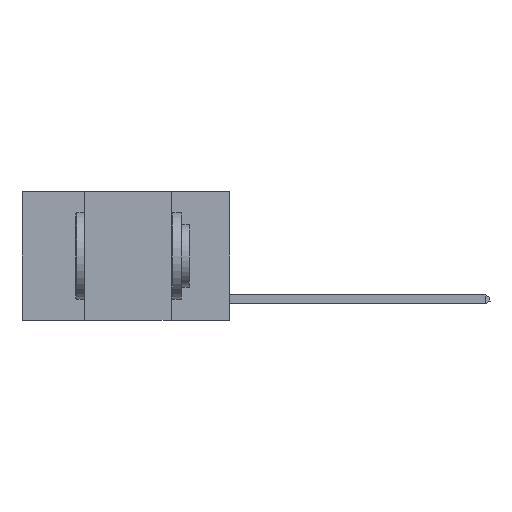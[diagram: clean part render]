
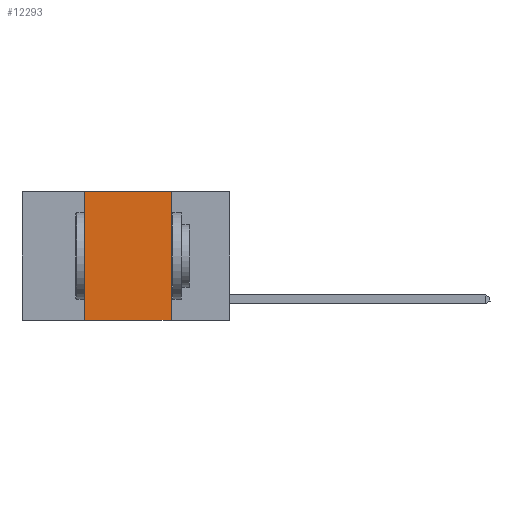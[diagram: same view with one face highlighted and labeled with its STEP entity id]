
A CAD part, left-side view. The second image highlights one B-rep face of the part: STEP entity #12293.
In plain terms, the highlighted planar face has unit normal (-1, 0, 0).
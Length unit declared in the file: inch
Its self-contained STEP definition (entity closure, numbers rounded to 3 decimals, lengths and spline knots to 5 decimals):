
#51 = AXIS2_PLACEMENT_3D ( 'NONE', #11276, #17470, #3569 ) ;
#1092 = CARTESIAN_POINT ( 'NONE',  ( 0., 0.42, 0. ) ) ;
#1306 = EDGE_CURVE ( 'NONE', #6774, #16200, #11847, .T. ) ;
#1588 = EDGE_CURVE ( 'NONE', #6774, #11793, #8910, .T. ) ;
#1649 = PLANE ( 'NONE',  #51 ) ;
#3271 = VECTOR ( 'NONE', #3595, 39.37008 ) ;
#3569 = DIRECTION ( 'NONE',  ( 0., 0., -1. ) ) ;
#3595 = DIRECTION ( 'NONE',  ( 0., 0., -1. ) ) ;
#4987 = CARTESIAN_POINT ( 'NONE',  ( 0., 0.17, -0.37 ) ) ;
#6774 = VERTEX_POINT ( 'NONE', #12183 ) ;
#6800 = ORIENTED_EDGE ( 'NONE', *, *, #1588, .T. ) ;
#6830 = VECTOR ( 'NONE', #11538, 39.37008 ) ;
#6855 = EDGE_CURVE ( 'NONE', #16200, #14285, #7147, .T. ) ;
#7147 = LINE ( 'NONE', #11908, #17987 ) ;
#8768 = ORIENTED_EDGE ( 'NONE', *, *, #6855, .F. ) ;
#8910 = LINE ( 'NONE', #18463, #17835 ) ;
#11276 = CARTESIAN_POINT ( 'NONE',  ( 0., 0.6, 0. ) ) ;
#11538 = DIRECTION ( 'NONE',  ( 0., 0., 1. ) ) ;
#11661 = ORIENTED_EDGE ( 'NONE', *, *, #11863, .F. ) ;
#11793 = VERTEX_POINT ( 'NONE', #4987 ) ;
#11800 = DIRECTION ( 'NONE',  ( 0., -1., 0. ) ) ;
#11847 = LINE ( 'NONE', #1092, #6830 ) ;
#11863 = EDGE_CURVE ( 'NONE', #14285, #11793, #12642, .T. ) ;
#11908 = CARTESIAN_POINT ( 'NONE',  ( 0., 0.6, 0. ) ) ;
#12183 = CARTESIAN_POINT ( 'NONE',  ( 0., 0.42, -0.37 ) ) ;
#12293 = ADVANCED_FACE ( 'NONE', ( #18964 ), #1649, .F. ) ;
#12642 = LINE ( 'NONE', #18803, #3271 ) ;
#12670 = EDGE_LOOP ( 'NONE', ( #11661, #8768, #18224, #6800 ) ) ;
#14285 = VERTEX_POINT ( 'NONE', #14916 ) ;
#14916 = CARTESIAN_POINT ( 'NONE',  ( 0., 0.17, 0. ) ) ;
#16200 = VERTEX_POINT ( 'NONE', #18247 ) ;
#17470 = DIRECTION ( 'NONE',  ( 1., 0., 0. ) ) ;
#17835 = VECTOR ( 'NONE', #18354, 39.37008 ) ;
#17987 = VECTOR ( 'NONE', #11800, 39.37008 ) ;
#18224 = ORIENTED_EDGE ( 'NONE', *, *, #1306, .F. ) ;
#18247 = CARTESIAN_POINT ( 'NONE',  ( 0., 0.42, 0. ) ) ;
#18354 = DIRECTION ( 'NONE',  ( 0., -1., 0. ) ) ;
#18463 = CARTESIAN_POINT ( 'NONE',  ( 0., 0.6, -0.37 ) ) ;
#18803 = CARTESIAN_POINT ( 'NONE',  ( 0., 0.17, 0. ) ) ;
#18964 = FACE_OUTER_BOUND ( 'NONE', #12670, .T. ) ;
